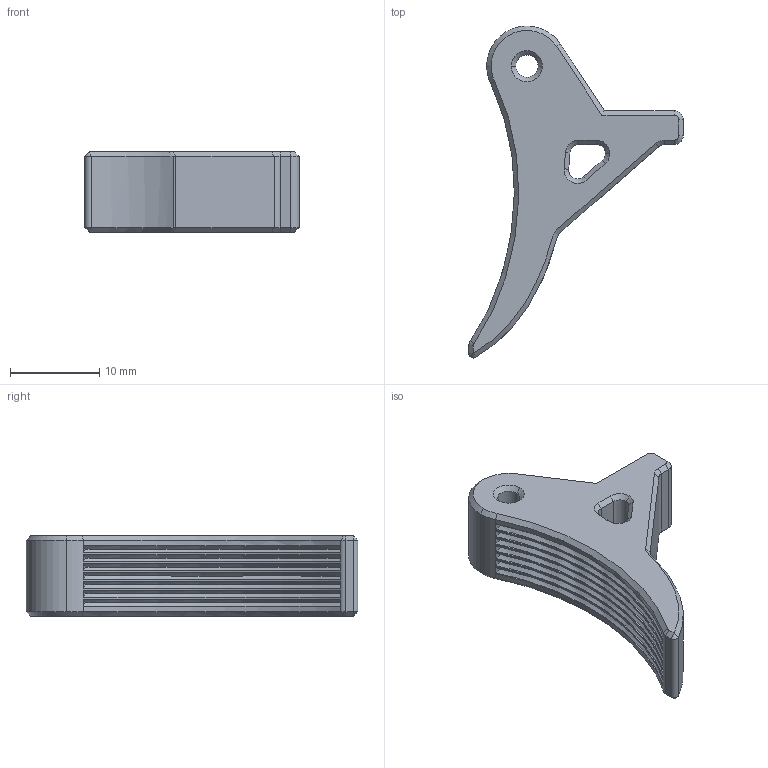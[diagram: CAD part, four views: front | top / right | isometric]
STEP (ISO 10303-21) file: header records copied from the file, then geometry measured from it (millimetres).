
FILE_DESCRIPTION (( 'STEP AP214' ), '1' );
FILE_NAME ('Trigger_V4.STEP', '2025-07-07T03:52:23', ( '' ), ( '' ), 'SwSTEP 2.0', 'SolidWorks 2020', '' );
FILE_SCHEMA (( 'AUTOMOTIVE_DESIGN' ));
Length unit declared in the file: millimetre
Products named in the file (1): Trigger_V4
Bounding box: 24 x 37.16 x 9 mm (x, y, z)
Volume: 2713.7 mm3; surface area: 1767.6 mm2
Topology: 1 solids, 1 shells, 139 faces, 335 edges, 196 vertices
Faces by surface type: plane 68, bspline 30, cone 27, cylinder 14
Entity records: 10223 total; most frequent: CARTESIAN_POINT 7217, ORIENTED_EDGE 666, DIRECTION 520, EDGE_CURVE 333, VERTEX_POINT 196, VECTOR 192, LINE 192, AXIS2_PLACEMENT_3D 164
